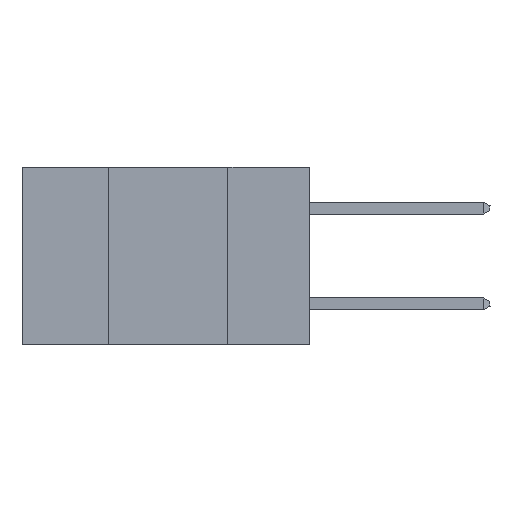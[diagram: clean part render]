
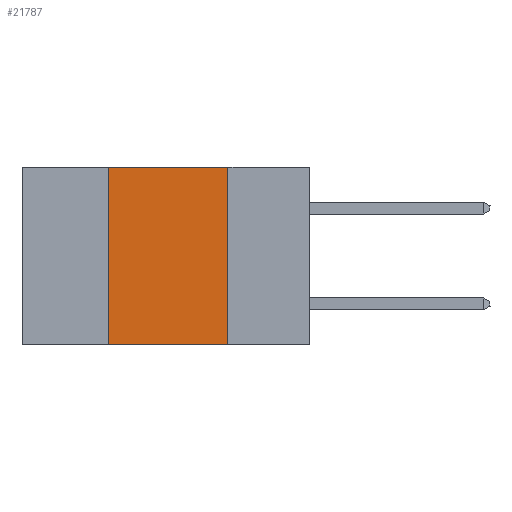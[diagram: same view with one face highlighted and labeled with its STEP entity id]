
A CAD part, left-side view. The second image highlights one B-rep face of the part: STEP entity #21787.
In plain terms, the highlighted planar face has unit normal (-1, 0, 0).
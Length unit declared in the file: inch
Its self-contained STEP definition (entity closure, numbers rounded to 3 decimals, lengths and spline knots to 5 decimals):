
#694 = LINE ( 'NONE', #10368, #10799 ) ;
#1306 = CARTESIAN_POINT ( 'NONE',  ( 0., 0.17, 0. ) ) ;
#1434 = AXIS2_PLACEMENT_3D ( 'NONE', #2876, #6483, #19723 ) ;
#2209 = VERTEX_POINT ( 'NONE', #20428 ) ;
#2876 = CARTESIAN_POINT ( 'NONE',  ( 0., 0.6, 0. ) ) ;
#2893 = LINE ( 'NONE', #20350, #23905 ) ;
#3559 = DIRECTION ( 'NONE',  ( 0., -1., 0. ) ) ;
#3623 = VERTEX_POINT ( 'NONE', #1306 ) ;
#4119 = EDGE_CURVE ( 'NONE', #3623, #2209, #2893, .T. ) ;
#4215 = LINE ( 'NONE', #14968, #19312 ) ;
#4595 = PLANE ( 'NONE',  #1434 ) ;
#6173 = EDGE_CURVE ( 'NONE', #15083, #2209, #4215, .T. ) ;
#6483 = DIRECTION ( 'NONE',  ( 1., 0., 0. ) ) ;
#6950 = ORIENTED_EDGE ( 'NONE', *, *, #10082, .F. ) ;
#7883 = VECTOR ( 'NONE', #23514, 39.37008 ) ;
#8477 = LINE ( 'NONE', #20020, #7883 ) ;
#8975 = FACE_OUTER_BOUND ( 'NONE', #16031, .T. ) ;
#9291 = ORIENTED_EDGE ( 'NONE', *, *, #4119, .F. ) ;
#10082 = EDGE_CURVE ( 'NONE', #15083, #14469, #8477, .T. ) ;
#10368 = CARTESIAN_POINT ( 'NONE',  ( 0., 0.6, 0. ) ) ;
#10799 = VECTOR ( 'NONE', #15716, 39.37008 ) ;
#12942 = ORIENTED_EDGE ( 'NONE', *, *, #14246, .F. ) ;
#14246 = EDGE_CURVE ( 'NONE', #14469, #3623, #694, .T. ) ;
#14469 = VERTEX_POINT ( 'NONE', #18018 ) ;
#14968 = CARTESIAN_POINT ( 'NONE',  ( 0., 0.6, -0.37 ) ) ;
#15083 = VERTEX_POINT ( 'NONE', #23808 ) ;
#15716 = DIRECTION ( 'NONE',  ( 0., -1., 0. ) ) ;
#16031 = EDGE_LOOP ( 'NONE', ( #9291, #12942, #6950, #19431 ) ) ;
#18018 = CARTESIAN_POINT ( 'NONE',  ( 0., 0.42, 0. ) ) ;
#19078 = DIRECTION ( 'NONE',  ( 0., 0., -1. ) ) ;
#19312 = VECTOR ( 'NONE', #3559, 39.37008 ) ;
#19431 = ORIENTED_EDGE ( 'NONE', *, *, #6173, .T. ) ;
#19723 = DIRECTION ( 'NONE',  ( 0., 0., -1. ) ) ;
#20020 = CARTESIAN_POINT ( 'NONE',  ( 0., 0.42, 0. ) ) ;
#20350 = CARTESIAN_POINT ( 'NONE',  ( 0., 0.17, 0. ) ) ;
#20428 = CARTESIAN_POINT ( 'NONE',  ( 0., 0.17, -0.37 ) ) ;
#21787 = ADVANCED_FACE ( 'NONE', ( #8975 ), #4595, .F. ) ;
#23514 = DIRECTION ( 'NONE',  ( 0., 0., 1. ) ) ;
#23808 = CARTESIAN_POINT ( 'NONE',  ( 0., 0.42, -0.37 ) ) ;
#23905 = VECTOR ( 'NONE', #19078, 39.37008 ) ;
